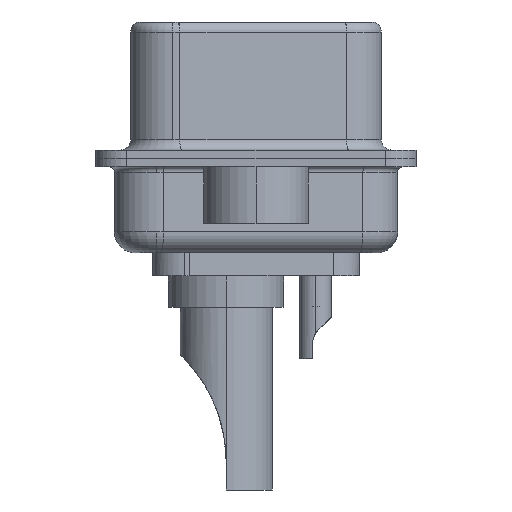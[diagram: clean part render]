
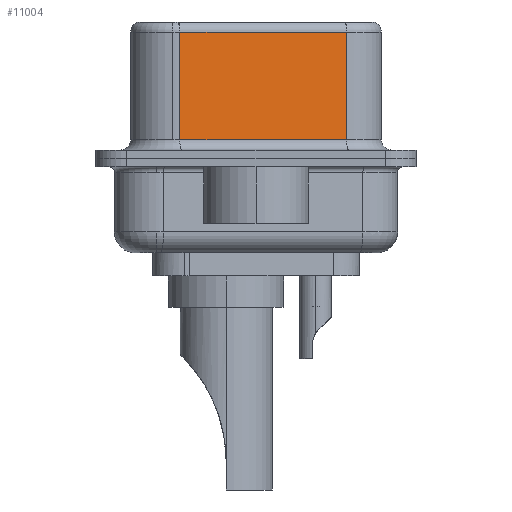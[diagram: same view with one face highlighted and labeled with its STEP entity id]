
A CAD part, left-side view. The second image highlights one B-rep face of the part: STEP entity #11004.
In plain terms, the highlighted planar face has unit normal (-0.985, -0.174, 0).
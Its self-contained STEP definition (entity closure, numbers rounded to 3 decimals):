
#226 = CARTESIAN_POINT ( 'NONE',  ( 5.132, -4.322, 6.52 ) ) ;
#492 = EDGE_CURVE ( 'NONE', #16762, #17332, #6222, .T. ) ;
#750 = VECTOR ( 'NONE', #6505, 1000. ) ;
#1236 = CARTESIAN_POINT ( 'NONE',  ( 3.73, 3.628, 0.9 ) ) ;
#2525 = FACE_OUTER_BOUND ( 'NONE', #15097, .T. ) ;
#3284 = CARTESIAN_POINT ( 'NONE',  ( 5.132, -4.322, 6.02 ) ) ;
#5089 = AXIS2_PLACEMENT_3D ( 'NONE', #9517, #23864, #11643 ) ;
#6011 = EDGE_CURVE ( 'NONE', #16762, #12092, #11461, .T. ) ;
#6222 = LINE ( 'NONE', #226, #750 ) ;
#6505 = DIRECTION ( 'NONE',  ( 0., 0., -1. ) ) ;
#7498 = EDGE_CURVE ( 'NONE', #22841, #17332, #24169, .T. ) ;
#9232 = CARTESIAN_POINT ( 'NONE',  ( 5.132, -4.322, 0.9 ) ) ;
#9517 = CARTESIAN_POINT ( 'NONE',  ( 5.132, -4.322, 6.52 ) ) ;
#11004 = ADVANCED_FACE ( 'NONE', ( #2525 ), #21780, .F. ) ;
#11461 = LINE ( 'NONE', #22530, #22305 ) ;
#11643 = DIRECTION ( 'NONE',  ( -0.174, 0.985, 0. ) ) ;
#12092 = VERTEX_POINT ( 'NONE', #12531 ) ;
#12468 = ORIENTED_EDGE ( 'NONE', *, *, #7498, .T. ) ;
#12531 = CARTESIAN_POINT ( 'NONE',  ( 3.73, 3.628, 6.02 ) ) ;
#13359 = VECTOR ( 'NONE', #19670, 1000. ) ;
#13373 = DIRECTION ( 'NONE',  ( 0., 0., -1. ) ) ;
#15097 = EDGE_LOOP ( 'NONE', ( #25898, #23154, #15557, #12468 ) ) ;
#15325 = VECTOR ( 'NONE', #13373, 1000. ) ;
#15557 = ORIENTED_EDGE ( 'NONE', *, *, #18505, .T. ) ;
#16762 = VERTEX_POINT ( 'NONE', #3284 ) ;
#17332 = VERTEX_POINT ( 'NONE', #9232 ) ;
#18505 = EDGE_CURVE ( 'NONE', #12092, #22841, #20658, .T. ) ;
#19670 = DIRECTION ( 'NONE',  ( 0.174, -0.985, 0. ) ) ;
#20658 = LINE ( 'NONE', #21418, #15325 ) ;
#20865 = CARTESIAN_POINT ( 'NONE',  ( 5.132, -4.322, 0.9 ) ) ;
#21260 = DIRECTION ( 'NONE',  ( -0.174, 0.985, 0. ) ) ;
#21418 = CARTESIAN_POINT ( 'NONE',  ( 3.73, 3.628, 6.52 ) ) ;
#21780 = PLANE ( 'NONE',  #5089 ) ;
#22305 = VECTOR ( 'NONE', #21260, 1000. ) ;
#22530 = CARTESIAN_POINT ( 'NONE',  ( 5.132, -4.322, 6.02 ) ) ;
#22841 = VERTEX_POINT ( 'NONE', #1236 ) ;
#23154 = ORIENTED_EDGE ( 'NONE', *, *, #6011, .T. ) ;
#23864 = DIRECTION ( 'NONE',  ( 0.985, 0.174, 0. ) ) ;
#24169 = LINE ( 'NONE', #20865, #13359 ) ;
#25898 = ORIENTED_EDGE ( 'NONE', *, *, #492, .F. ) ;
